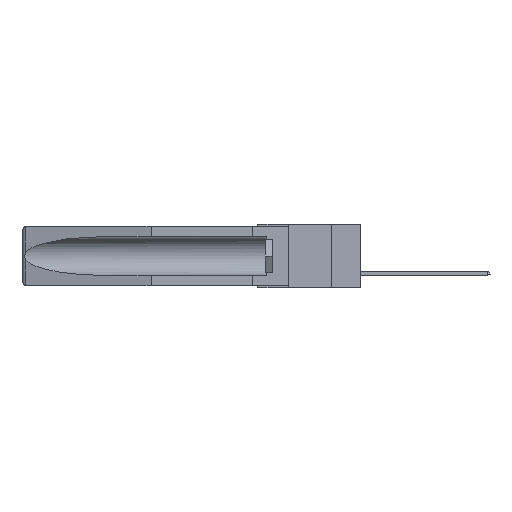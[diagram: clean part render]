
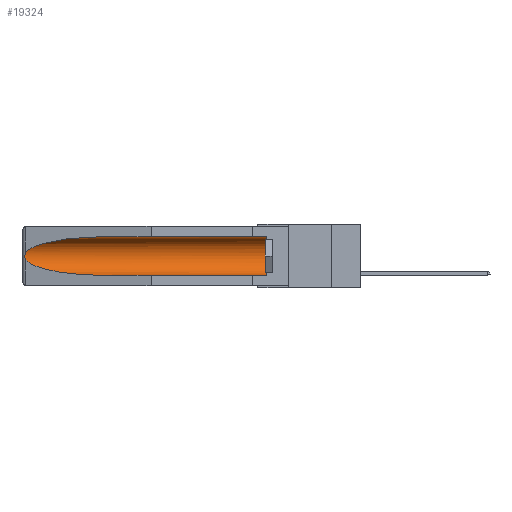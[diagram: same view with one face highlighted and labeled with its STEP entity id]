
A CAD part, left-side view. The second image highlights one B-rep face of the part: STEP entity #19324.
In plain terms, the highlighted cylindrical face has radius 2.857 mm (diameter 5.715 mm), a partial arc.
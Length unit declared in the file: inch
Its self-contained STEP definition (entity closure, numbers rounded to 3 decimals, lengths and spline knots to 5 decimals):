
#873 = EDGE_LOOP ( 'NONE', ( #19456, #14854, #20129, #1264, #9285, #2624 ) ) ;
#890 = CIRCLE ( 'NONE', #967, 0.1125 ) ;
#967 = AXIS2_PLACEMENT_3D ( 'NONE', #13858, #17072, #5937 ) ;
#1264 = ORIENTED_EDGE ( 'NONE', *, *, #15439, .F. ) ;
#1785 = CARTESIAN_POINT ( 'NONE',  ( 0.26654, 1.53092, -0.15636 ) ) ;
#2230 = VECTOR ( 'NONE', #17754, 39.37008 ) ;
#2624 = ORIENTED_EDGE ( 'NONE', *, *, #5058, .T. ) ;
#2651 =( BOUNDED_CURVE ( )  B_SPLINE_CURVE ( 3, ( #9714, #17636, #16200, #4143 ),
 .UNSPECIFIED., .F., .F. ) 
 B_SPLINE_CURVE_WITH_KNOTS ( ( 4, 4 ),
 ( 0.1948, 1.5708 ),
 .UNSPECIFIED. ) 
 CURVE ( )  GEOMETRIC_REPRESENTATION_ITEM ( )  RATIONAL_B_SPLINE_CURVE ( ( 1., 0.848, 0.848, 1. ) ) 
 REPRESENTATION_ITEM ( '' )  );
#3398 = CARTESIAN_POINT ( 'NONE',  ( 0.26537, 1.52718, -0.19328 ) ) ;
#3836 = VERTEX_POINT ( 'NONE', #12943 ) ;
#4143 = CARTESIAN_POINT ( 'NONE',  ( 0.155, 1.07973, -0.284 ) ) ;
#5058 = EDGE_CURVE ( 'NONE', #10745, #7222, #15003, .T. ) ;
#5377 = CARTESIAN_POINT ( 'NONE',  ( 0.155, -0.30754, -0.284 ) ) ;
#5423 = CARTESIAN_POINT ( 'NONE',  ( 0.21114, 1.30732, -0.059 ) ) ;
#5645 = B_SPLINE_CURVE_WITH_KNOTS ( 'NONE', 3,
 ( #9781, #9636, #1785, #12670, #12805, #15987, #12875, #17485, #9505, #3398 ),
 .UNSPECIFIED., .F., .F.,
 ( 4, 2, 2, 2, 4 ),
 ( 0., 0.00029, 0.00058, 0.00087, 0.00117 ),
 .UNSPECIFIED. ) ;
#5937 = DIRECTION ( 'NONE',  ( 0., 0., 1. ) ) ;
#6207 = CARTESIAN_POINT ( 'NONE',  ( 0.155, -0.30754, -0.1715 ) ) ;
#6635 = CARTESIAN_POINT ( 'NONE',  ( 0.155, 0.126, -0.284 ) ) ;
#7222 = VERTEX_POINT ( 'NONE', #19562 ) ;
#7740 = CARTESIAN_POINT ( 'NONE',  ( 0.155, -0.30754, -0.059 ) ) ;
#7803 = DIRECTION ( 'NONE',  ( 0., 1., 0. ) ) ;
#8106 = CARTESIAN_POINT ( 'NONE',  ( 0.155, 0.126, -0.059 ) ) ;
#8988 = CARTESIAN_POINT ( 'NONE',  ( 0.26537, 1.52718, -0.19328 ) ) ;
#9178 = CYLINDRICAL_SURFACE ( 'NONE', #11552, 0.1125 ) ;
#9242 = DIRECTION ( 'NONE',  ( 0., 1., 0. ) ) ;
#9285 = ORIENTED_EDGE ( 'NONE', *, *, #11554, .T. ) ;
#9505 = CARTESIAN_POINT ( 'NONE',  ( 0.26597, 1.5296, -0.19026 ) ) ;
#9636 = CARTESIAN_POINT ( 'NONE',  ( 0.26597, 1.52961, -0.15275 ) ) ;
#9714 = CARTESIAN_POINT ( 'NONE',  ( 0.26537, 1.52718, -0.19328 ) ) ;
#9717 = CARTESIAN_POINT ( 'NONE',  ( 0.26537, 1.52718, -0.14972 ) ) ;
#9781 = CARTESIAN_POINT ( 'NONE',  ( 0.26537, 1.52718, -0.14972 ) ) ;
#10745 = VERTEX_POINT ( 'NONE', #8106 ) ;
#11552 = AXIS2_PLACEMENT_3D ( 'NONE', #6207, #9242, #12328 ) ;
#11554 = EDGE_CURVE ( 'NONE', #18333, #10745, #890, .T. ) ;
#11610 = VERTEX_POINT ( 'NONE', #9717 ) ;
#12103 = VERTEX_POINT ( 'NONE', #8988 ) ;
#12328 = DIRECTION ( 'NONE',  ( 0., 0., 1. ) ) ;
#12670 = CARTESIAN_POINT ( 'NONE',  ( 0.2673, 1.5327, -0.16383 ) ) ;
#12805 = CARTESIAN_POINT ( 'NONE',  ( 0.2675, 1.53308, -0.16763 ) ) ;
#12875 = CARTESIAN_POINT ( 'NONE',  ( 0.2673, 1.53269, -0.17917 ) ) ;
#12943 = CARTESIAN_POINT ( 'NONE',  ( 0.155, 1.07973, -0.284 ) ) ;
#13858 = CARTESIAN_POINT ( 'NONE',  ( 0.155, 0.126, -0.1715 ) ) ;
#14356 = FACE_OUTER_BOUND ( 'NONE', #873, .T. ) ;
#14756 = LINE ( 'NONE', #5377, #2230 ) ;
#14854 = ORIENTED_EDGE ( 'NONE', *, *, #19458, .T. ) ;
#14916 = CARTESIAN_POINT ( 'NONE',  ( 0.155, 1.07973, -0.059 ) ) ;
#15003 = LINE ( 'NONE', #7740, #19454 ) ;
#15439 = EDGE_CURVE ( 'NONE', #18333, #3836, #14756, .T. ) ;
#15987 = CARTESIAN_POINT ( 'NONE',  ( 0.2675, 1.53308, -0.17534 ) ) ;
#16200 = CARTESIAN_POINT ( 'NONE',  ( 0.21114, 1.30732, -0.284 ) ) ;
#16437 = CARTESIAN_POINT ( 'NONE',  ( 0.25451, 1.48313, -0.09465 ) ) ;
#17072 = DIRECTION ( 'NONE',  ( 0., -1., 0. ) ) ;
#17485 = CARTESIAN_POINT ( 'NONE',  ( 0.26655, 1.53094, -0.18657 ) ) ;
#17636 = CARTESIAN_POINT ( 'NONE',  ( 0.25451, 1.48313, -0.24835 ) ) ;
#17754 = DIRECTION ( 'NONE',  ( 0., 1., 0. ) ) ;
#17998 = CARTESIAN_POINT ( 'NONE',  ( 0.26537, 1.52718, -0.14972 ) ) ;
#18333 = VERTEX_POINT ( 'NONE', #6635 ) ;
#19324 = ADVANCED_FACE ( 'NONE', ( #14356 ), #9178, .F. ) ;
#19454 = VECTOR ( 'NONE', #7803, 39.37008 ) ;
#19456 = ORIENTED_EDGE ( 'NONE', *, *, #19519, .T. ) ;
#19458 = EDGE_CURVE ( 'NONE', #11610, #12103, #5645, .T. ) ;
#19519 = EDGE_CURVE ( 'NONE', #7222, #11610, #20286, .T. ) ;
#19562 = CARTESIAN_POINT ( 'NONE',  ( 0.155, 1.07973, -0.059 ) ) ;
#20077 = EDGE_CURVE ( 'NONE', #12103, #3836, #2651, .T. ) ;
#20129 = ORIENTED_EDGE ( 'NONE', *, *, #20077, .T. ) ;
#20286 =( BOUNDED_CURVE ( )  B_SPLINE_CURVE ( 3, ( #14916, #5423, #16437, #17998 ),
 .UNSPECIFIED., .F., .T. ) 
 B_SPLINE_CURVE_WITH_KNOTS ( ( 4, 4 ),
 ( 4.71239, 6.08839 ),
 .UNSPECIFIED. ) 
 CURVE ( )  GEOMETRIC_REPRESENTATION_ITEM ( )  RATIONAL_B_SPLINE_CURVE ( ( 1., 0.848, 0.848, 1. ) ) 
 REPRESENTATION_ITEM ( '' )  );
